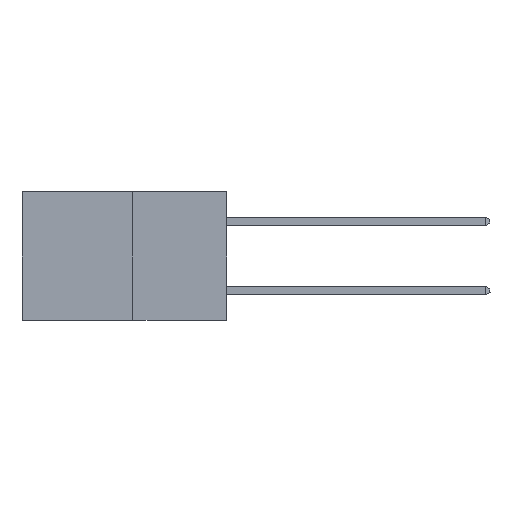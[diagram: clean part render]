
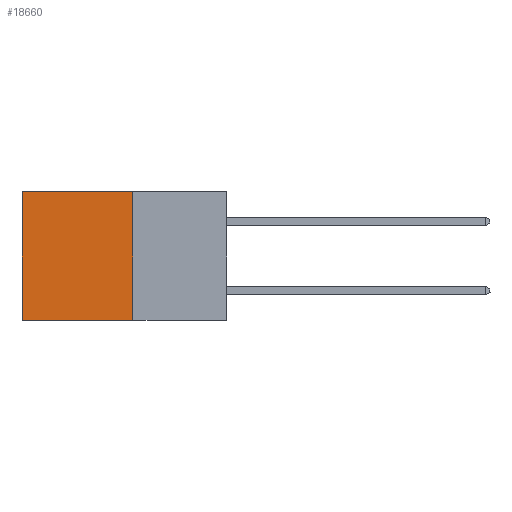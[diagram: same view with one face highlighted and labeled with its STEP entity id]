
A CAD part, left-side view. The second image highlights one B-rep face of the part: STEP entity #18660.
In plain terms, the highlighted planar face has unit normal (-1, 0, 0).
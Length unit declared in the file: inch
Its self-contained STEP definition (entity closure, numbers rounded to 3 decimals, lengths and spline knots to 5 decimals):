
#668 = CARTESIAN_POINT ( 'NONE',  ( 0.277, 0.27, -0.37 ) ) ;
#698 = CARTESIAN_POINT ( 'NONE',  ( 0.277, 0.59, 0. ) ) ;
#1111 = VECTOR ( 'NONE', #13485, 39.37008 ) ;
#1990 = DIRECTION ( 'NONE',  ( 0., 0., -1. ) ) ;
#2477 = VECTOR ( 'NONE', #7853, 39.37008 ) ;
#2736 = ORIENTED_EDGE ( 'NONE', *, *, #21797, .F. ) ;
#4211 = PLANE ( 'NONE',  #15935 ) ;
#5001 = VERTEX_POINT ( 'NONE', #14500 ) ;
#5768 = DIRECTION ( 'NONE',  ( 0., 1., 0. ) ) ;
#6598 = VERTEX_POINT ( 'NONE', #698 ) ;
#7697 = DIRECTION ( 'NONE',  ( 0., 0., -1. ) ) ;
#7853 = DIRECTION ( 'NONE',  ( 0., 1., 0. ) ) ;
#10454 = EDGE_CURVE ( 'NONE', #6598, #25062, #14129, .T. ) ;
#10725 = ORIENTED_EDGE ( 'NONE', *, *, #28226, .F. ) ;
#11809 = VECTOR ( 'NONE', #7697, 39.37008 ) ;
#13485 = DIRECTION ( 'NONE',  ( 0., 0., -1. ) ) ;
#13730 = VECTOR ( 'NONE', #5768, 39.37008 ) ;
#14129 = LINE ( 'NONE', #24868, #1111 ) ;
#14500 = CARTESIAN_POINT ( 'NONE',  ( 0.277, 0.27, -0.37 ) ) ;
#15817 = DIRECTION ( 'NONE',  ( 1., 0., 0. ) ) ;
#15935 = AXIS2_PLACEMENT_3D ( 'NONE', #29427, #15817, #1990 ) ;
#17989 = EDGE_LOOP ( 'NONE', ( #25370, #10725, #2736, #22535 ) ) ;
#18610 = LINE ( 'NONE', #668, #11809 ) ;
#18660 = ADVANCED_FACE ( 'NONE', ( #25884 ), #4211, .F. ) ;
#19265 = CARTESIAN_POINT ( 'NONE',  ( 0.277, 0.27, -0.37 ) ) ;
#19752 = VERTEX_POINT ( 'NONE', #28485 ) ;
#19795 = LINE ( 'NONE', #26311, #13730 ) ;
#21572 = LINE ( 'NONE', #19265, #2477 ) ;
#21797 = EDGE_CURVE ( 'NONE', #19752, #5001, #18610, .T. ) ;
#22535 = ORIENTED_EDGE ( 'NONE', *, *, #26941, .T. ) ;
#24868 = CARTESIAN_POINT ( 'NONE',  ( 0.277, 0.59, -0.37 ) ) ;
#25062 = VERTEX_POINT ( 'NONE', #27685 ) ;
#25370 = ORIENTED_EDGE ( 'NONE', *, *, #10454, .T. ) ;
#25884 = FACE_OUTER_BOUND ( 'NONE', #17989, .T. ) ;
#26311 = CARTESIAN_POINT ( 'NONE',  ( 0.277, 0.27, 0. ) ) ;
#26941 = EDGE_CURVE ( 'NONE', #19752, #6598, #19795, .T. ) ;
#27685 = CARTESIAN_POINT ( 'NONE',  ( 0.277, 0.59, -0.37 ) ) ;
#28226 = EDGE_CURVE ( 'NONE', #5001, #25062, #21572, .T. ) ;
#28485 = CARTESIAN_POINT ( 'NONE',  ( 0.277, 0.27, 0. ) ) ;
#29427 = CARTESIAN_POINT ( 'NONE',  ( 0.277, 0.27, -0.37 ) ) ;
